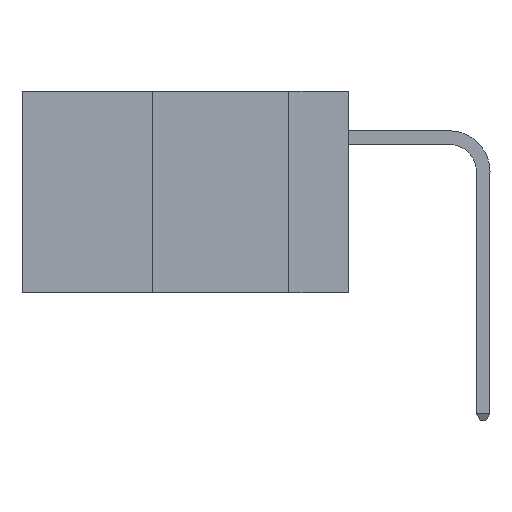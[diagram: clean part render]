
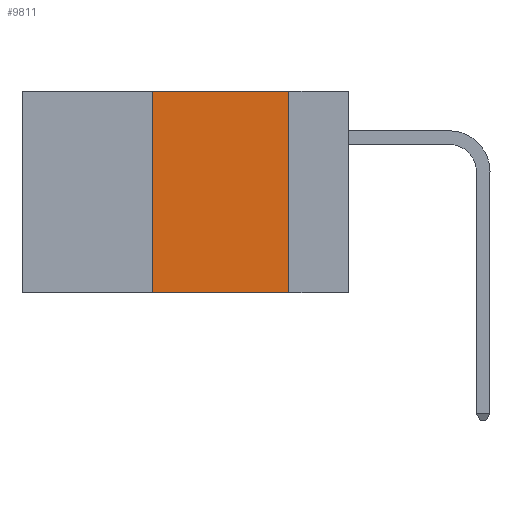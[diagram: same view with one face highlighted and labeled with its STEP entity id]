
A CAD part, left-side view. The second image highlights one B-rep face of the part: STEP entity #9811.
In plain terms, the highlighted planar face has unit normal (-1, 0, 0).
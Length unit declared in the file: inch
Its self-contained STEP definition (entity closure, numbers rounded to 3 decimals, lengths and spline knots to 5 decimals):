
#764 = AXIS2_PLACEMENT_3D ( 'NONE', #2712, #10675, #6672 ) ;
#925 = CARTESIAN_POINT ( 'NONE',  ( 0., 0.36, 0. ) ) ;
#1504 = VECTOR ( 'NONE', #5685, 39.37008 ) ;
#1606 = LINE ( 'NONE', #4744, #1504 ) ;
#1659 = CARTESIAN_POINT ( 'NONE',  ( 0., 0.11, -0.37 ) ) ;
#1836 = VECTOR ( 'NONE', #4702, 39.37008 ) ;
#1902 = LINE ( 'NONE', #3700, #1836 ) ;
#2059 = CARTESIAN_POINT ( 'NONE',  ( 0., 0.11, 0. ) ) ;
#2286 = CARTESIAN_POINT ( 'NONE',  ( 0., 0.36, -0.37 ) ) ;
#2687 = LINE ( 'NONE', #10473, #7515 ) ;
#2712 = CARTESIAN_POINT ( 'NONE',  ( 0., 0.6, 0. ) ) ;
#3073 = EDGE_LOOP ( 'NONE', ( #10159, #10238, #9188, #8863 ) ) ;
#3567 = EDGE_CURVE ( 'NONE', #6349, #10063, #6558, .T. ) ;
#3700 = CARTESIAN_POINT ( 'NONE',  ( 0., 0.6, -0.37 ) ) ;
#4702 = DIRECTION ( 'NONE',  ( 0., -1., 0. ) ) ;
#4744 = CARTESIAN_POINT ( 'NONE',  ( 0., 0.36, 0. ) ) ;
#5412 = DIRECTION ( 'NONE',  ( 0., 0., -1. ) ) ;
#5685 = DIRECTION ( 'NONE',  ( 0., 0., 1. ) ) ;
#5836 = CARTESIAN_POINT ( 'NONE',  ( 0., 0.6, 0. ) ) ;
#5837 = DIRECTION ( 'NONE',  ( 0., -1., 0. ) ) ;
#5996 = EDGE_CURVE ( 'NONE', #10063, #10424, #2687, .T. ) ;
#6106 = EDGE_CURVE ( 'NONE', #9541, #10424, #1902, .T. ) ;
#6122 = EDGE_CURVE ( 'NONE', #9541, #6349, #1606, .T. ) ;
#6349 = VERTEX_POINT ( 'NONE', #925 ) ;
#6558 = LINE ( 'NONE', #5836, #6739 ) ;
#6672 = DIRECTION ( 'NONE',  ( 0., 0., -1. ) ) ;
#6739 = VECTOR ( 'NONE', #5837, 39.37008 ) ;
#7515 = VECTOR ( 'NONE', #5412, 39.37008 ) ;
#8863 = ORIENTED_EDGE ( 'NONE', *, *, #6106, .T. ) ;
#9188 = ORIENTED_EDGE ( 'NONE', *, *, #6122, .F. ) ;
#9541 = VERTEX_POINT ( 'NONE', #2286 ) ;
#9781 = FACE_OUTER_BOUND ( 'NONE', #3073, .T. ) ;
#9811 = ADVANCED_FACE ( 'NONE', ( #9781 ), #10105, .F. ) ;
#10063 = VERTEX_POINT ( 'NONE', #2059 ) ;
#10105 = PLANE ( 'NONE',  #764 ) ;
#10159 = ORIENTED_EDGE ( 'NONE', *, *, #5996, .F. ) ;
#10238 = ORIENTED_EDGE ( 'NONE', *, *, #3567, .F. ) ;
#10424 = VERTEX_POINT ( 'NONE', #1659 ) ;
#10473 = CARTESIAN_POINT ( 'NONE',  ( 0., 0.11, 0. ) ) ;
#10675 = DIRECTION ( 'NONE',  ( 1., 0., 0. ) ) ;
